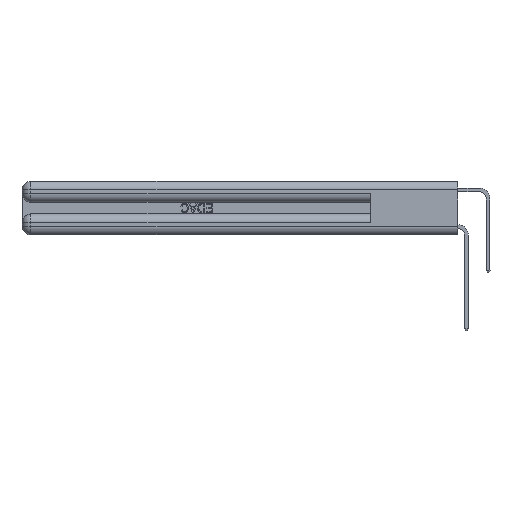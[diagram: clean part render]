
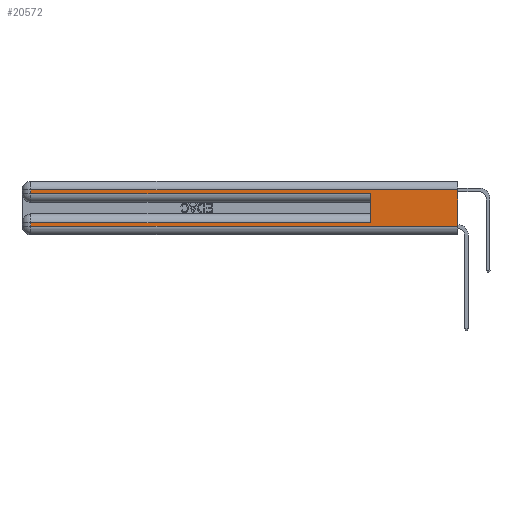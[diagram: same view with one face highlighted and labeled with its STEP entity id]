
A CAD part, left-side view. The second image highlights one B-rep face of the part: STEP entity #20572.
In plain terms, the highlighted planar face has unit normal (-1, 0, 0).
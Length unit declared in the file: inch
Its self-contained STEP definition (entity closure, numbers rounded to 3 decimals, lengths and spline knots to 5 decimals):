
#12 = LINE ( 'NONE', #21798, #21980 ) ;
#446 = CARTESIAN_POINT ( 'NONE',  ( 0., 0.6, 0.285 ) ) ;
#1284 = CARTESIAN_POINT ( 'NONE',  ( 0., 0., 0.31 ) ) ;
#2240 = EDGE_CURVE ( 'NONE', #22332, #20354, #12, .T. ) ;
#2375 = EDGE_CURVE ( 'NONE', #16005, #7007, #20364, .T. ) ;
#2840 = CARTESIAN_POINT ( 'NONE',  ( 0., 0., 0.37 ) ) ;
#3765 = EDGE_CURVE ( 'NONE', #20354, #23768, #20849, .T. ) ;
#4532 = ORIENTED_EDGE ( 'NONE', *, *, #2375, .T. ) ;
#4737 = ORIENTED_EDGE ( 'NONE', *, *, #27096, .F. ) ;
#4882 = DIRECTION ( 'NONE',  ( 0., 0., -1. ) ) ;
#4917 = VERTEX_POINT ( 'NONE', #15800 ) ;
#5044 = CARTESIAN_POINT ( 'NONE',  ( 0., 0.6, 0.085 ) ) ;
#5335 = VECTOR ( 'NONE', #24804, 39.37008 ) ;
#5526 = CARTESIAN_POINT ( 'NONE',  ( 0., 0., 0.31 ) ) ;
#5746 = VERTEX_POINT ( 'NONE', #446 ) ;
#5839 = PLANE ( 'NONE',  #24816 ) ;
#6114 = ORIENTED_EDGE ( 'NONE', *, *, #20020, .T. ) ;
#6464 = CARTESIAN_POINT ( 'NONE',  ( 0., 0., 0.085 ) ) ;
#6611 = LINE ( 'NONE', #6464, #27818 ) ;
#7007 = VERTEX_POINT ( 'NONE', #25375 ) ;
#7718 = CARTESIAN_POINT ( 'NONE',  ( 0., 0.6, 0.145 ) ) ;
#8572 = ORIENTED_EDGE ( 'NONE', *, *, #9461, .T. ) ;
#9355 = VECTOR ( 'NONE', #12574, 39.37008 ) ;
#9461 = EDGE_CURVE ( 'NONE', #7007, #4917, #23562, .T. ) ;
#9990 = LINE ( 'NONE', #11859, #16846 ) ;
#10247 = DIRECTION ( 'NONE',  ( 0., 0., -1. ) ) ;
#10314 = ORIENTED_EDGE ( 'NONE', *, *, #2240, .T. ) ;
#10682 = CARTESIAN_POINT ( 'NONE',  ( 0., 2.94, 0.085 ) ) ;
#11349 = DIRECTION ( 'NONE',  ( 0., -1., 0. ) ) ;
#11499 = CARTESIAN_POINT ( 'NONE',  ( 0., 2.94, 0.06 ) ) ;
#11859 = CARTESIAN_POINT ( 'NONE',  ( 0., 0., 0.285 ) ) ;
#12237 = LINE ( 'NONE', #24926, #24908 ) ;
#12457 = DIRECTION ( 'NONE',  ( 1., 0., 0. ) ) ;
#12519 = ORIENTED_EDGE ( 'NONE', *, *, #27833, .F. ) ;
#12574 = DIRECTION ( 'NONE',  ( 0., 0., 1. ) ) ;
#13229 = DIRECTION ( 'NONE',  ( 0., 1., 0. ) ) ;
#15800 = CARTESIAN_POINT ( 'NONE',  ( 0., 2.94, 0.285 ) ) ;
#16005 = VERTEX_POINT ( 'NONE', #1284 ) ;
#16573 = ORIENTED_EDGE ( 'NONE', *, *, #3765, .T. ) ;
#16846 = VECTOR ( 'NONE', #26740, 39.37008 ) ;
#17629 = DIRECTION ( 'NONE',  ( 0., 0., -1. ) ) ;
#17815 = CARTESIAN_POINT ( 'NONE',  ( 0., 0., 0.06 ) ) ;
#18774 = CARTESIAN_POINT ( 'NONE',  ( 0., 2.94, 0.37 ) ) ;
#19699 = LINE ( 'NONE', #7718, #9355 ) ;
#20020 = EDGE_CURVE ( 'NONE', #4917, #5746, #9990, .T. ) ;
#20354 = VERTEX_POINT ( 'NONE', #11499 ) ;
#20364 = LINE ( 'NONE', #5526, #5335 ) ;
#20480 = VECTOR ( 'NONE', #11349, 39.37008 ) ;
#20572 = ADVANCED_FACE ( 'NONE', ( #22263 ), #5839, .F. ) ;
#20849 = LINE ( 'NONE', #30334, #20480 ) ;
#21798 = CARTESIAN_POINT ( 'NONE',  ( 0., 2.94, 0.37 ) ) ;
#21980 = VECTOR ( 'NONE', #28910, 39.37008 ) ;
#22070 = EDGE_CURVE ( 'NONE', #25417, #22332, #6611, .T. ) ;
#22263 = FACE_OUTER_BOUND ( 'NONE', #28145, .T. ) ;
#22332 = VERTEX_POINT ( 'NONE', #10682 ) ;
#23562 = LINE ( 'NONE', #18774, #25409 ) ;
#23768 = VERTEX_POINT ( 'NONE', #17815 ) ;
#24804 = DIRECTION ( 'NONE',  ( 0., 1., 0. ) ) ;
#24816 = AXIS2_PLACEMENT_3D ( 'NONE', #2840, #12457, #10247 ) ;
#24908 = VECTOR ( 'NONE', #17629, 39.37008 ) ;
#24926 = CARTESIAN_POINT ( 'NONE',  ( 0., 0., 0.37 ) ) ;
#25375 = CARTESIAN_POINT ( 'NONE',  ( 0., 2.94, 0.31 ) ) ;
#25409 = VECTOR ( 'NONE', #4882, 39.37008 ) ;
#25417 = VERTEX_POINT ( 'NONE', #5044 ) ;
#26740 = DIRECTION ( 'NONE',  ( 0., -1., 0. ) ) ;
#27096 = EDGE_CURVE ( 'NONE', #25417, #5746, #19699, .T. ) ;
#27818 = VECTOR ( 'NONE', #13229, 39.37008 ) ;
#27833 = EDGE_CURVE ( 'NONE', #16005, #23768, #12237, .T. ) ;
#28145 = EDGE_LOOP ( 'NONE', ( #12519, #4532, #8572, #6114, #4737, #28660, #10314, #16573 ) ) ;
#28660 = ORIENTED_EDGE ( 'NONE', *, *, #22070, .T. ) ;
#28910 = DIRECTION ( 'NONE',  ( 0., 0., -1. ) ) ;
#30334 = CARTESIAN_POINT ( 'NONE',  ( 0., 0., 0.06 ) ) ;
